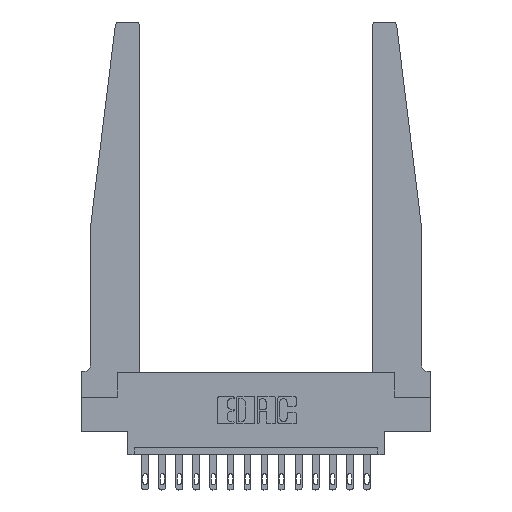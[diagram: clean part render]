
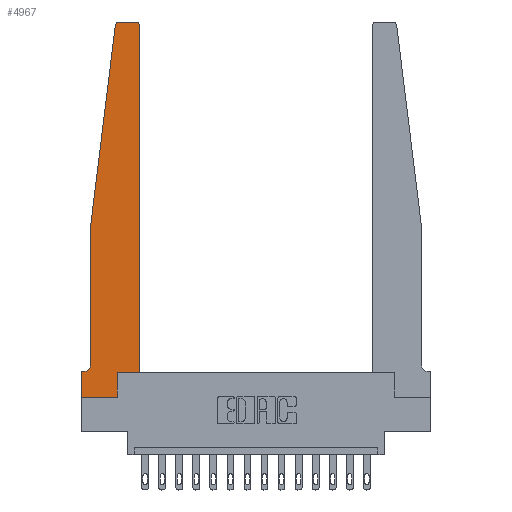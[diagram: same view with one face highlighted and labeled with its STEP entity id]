
A CAD part, top view. The second image highlights one B-rep face of the part: STEP entity #4967.
In plain terms, the highlighted planar face has unit normal (0, 0, 1).
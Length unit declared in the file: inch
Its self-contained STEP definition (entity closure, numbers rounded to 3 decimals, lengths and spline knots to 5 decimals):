
#178 = VERTEX_POINT ( 'NONE', #15564 ) ;
#372 = VERTEX_POINT ( 'NONE', #8095 ) ;
#437 = VERTEX_POINT ( 'NONE', #2567 ) ;
#461 = VERTEX_POINT ( 'NONE', #17534 ) ;
#1081 = VECTOR ( 'NONE', #7039, 39.37008 ) ;
#1116 = EDGE_CURVE ( 'NONE', #6186, #15797, #12551, .T. ) ;
#1315 = CARTESIAN_POINT ( 'NONE',  ( 0.015, 0.2375, 0.37 ) ) ;
#1372 = CARTESIAN_POINT ( 'NONE',  ( 0., 0., 0.37 ) ) ;
#1533 = ORIENTED_EDGE ( 'NONE', *, *, #12588, .T. ) ;
#1558 = DIRECTION ( 'NONE',  ( 0., -1., 0. ) ) ;
#1719 = VECTOR ( 'NONE', #12157, 39.37008 ) ;
#2425 = VERTEX_POINT ( 'NONE', #6968 ) ;
#2567 = CARTESIAN_POINT ( 'NONE',  ( 0.065, 1.25, 0.37 ) ) ;
#2598 = AXIS2_PLACEMENT_3D ( 'NONE', #13677, #2856, #17561 ) ;
#2856 = DIRECTION ( 'NONE',  ( 0., 0., 1. ) ) ;
#2908 = ORIENTED_EDGE ( 'NONE', *, *, #3953, .T. ) ;
#2912 = CARTESIAN_POINT ( 'NONE',  ( 0.395, 2.72, 0.37 ) ) ;
#2923 = DIRECTION ( 'NONE',  ( 0., 0., -1. ) ) ;
#2961 = EDGE_CURVE ( 'NONE', #10690, #16546, #6983, .T. ) ;
#3179 = VECTOR ( 'NONE', #1558, 39.37008 ) ;
#3345 = CARTESIAN_POINT ( 'NONE',  ( 0., 0., 0.37 ) ) ;
#3458 = VECTOR ( 'NONE', #15528, 39.37008 ) ;
#3953 = EDGE_CURVE ( 'NONE', #2425, #178, #16404, .T. ) ;
#4570 = CARTESIAN_POINT ( 'NONE',  ( 0., 0.1875, 0.37 ) ) ;
#4571 = EDGE_CURVE ( 'NONE', #437, #461, #13076, .T. ) ;
#4758 = EDGE_CURVE ( 'NONE', #12290, #11077, #11020, .T. ) ;
#4967 = ADVANCED_FACE ( 'NONE', ( #6512 ), #10468, .T. ) ;
#5254 = ORIENTED_EDGE ( 'NONE', *, *, #13176, .T. ) ;
#5280 = CARTESIAN_POINT ( 'NONE',  ( 0., 0.1875, 0.37 ) ) ;
#5446 = AXIS2_PLACEMENT_3D ( 'NONE', #5280, #10382, #9026 ) ;
#5924 = EDGE_LOOP ( 'NONE', ( #12108, #15944, #1533, #17374, #13289, #5254, #8734, #6416, #2908, #10328, #7662, #10372 ) ) ;
#6150 = CARTESIAN_POINT ( 'NONE',  ( 0.395, 2.75, 0.37 ) ) ;
#6186 = VERTEX_POINT ( 'NONE', #10662 ) ;
#6416 = ORIENTED_EDGE ( 'NONE', *, *, #7747, .T. ) ;
#6512 = FACE_OUTER_BOUND ( 'NONE', #5924, .T. ) ;
#6644 = DIRECTION ( 'NONE',  ( -1., 0., 0. ) ) ;
#6800 = VECTOR ( 'NONE', #15954, 39.37008 ) ;
#6968 = CARTESIAN_POINT ( 'NONE',  ( 0.2605, 0., 0.37 ) ) ;
#6983 = CIRCLE ( 'NONE', #17050, 0.03 ) ;
#6995 = EDGE_CURVE ( 'NONE', #16546, #6186, #8730, .T. ) ;
#7039 = DIRECTION ( 'NONE',  ( 0., 1., 0. ) ) ;
#7467 = CARTESIAN_POINT ( 'NONE',  ( 0.425, 0.18, 0.37 ) ) ;
#7662 = ORIENTED_EDGE ( 'NONE', *, *, #9104, .T. ) ;
#7747 = EDGE_CURVE ( 'NONE', #11077, #2425, #14326, .T. ) ;
#8095 = CARTESIAN_POINT ( 'NONE',  ( 0.015, 0.1875, 0.37 ) ) ;
#8730 = LINE ( 'NONE', #17008, #11979 ) ;
#8734 = ORIENTED_EDGE ( 'NONE', *, *, #4758, .T. ) ;
#9026 = DIRECTION ( 'NONE',  ( 1., 0., 0. ) ) ;
#9104 = EDGE_CURVE ( 'NONE', #15228, #10690, #15219, .T. ) ;
#9974 = VECTOR ( 'NONE', #13397, 39.37008 ) ;
#10060 = DIRECTION ( 'NONE',  ( -0.122, -0.992, 0. ) ) ;
#10076 = CARTESIAN_POINT ( 'NONE',  ( 0., 0., 0.37 ) ) ;
#10172 = CARTESIAN_POINT ( 'NONE',  ( 0.425, 2.72, 0.37 ) ) ;
#10328 = ORIENTED_EDGE ( 'NONE', *, *, #14896, .T. ) ;
#10372 = ORIENTED_EDGE ( 'NONE', *, *, #2961, .T. ) ;
#10382 = DIRECTION ( 'NONE',  ( 0., 0., 1. ) ) ;
#10468 = PLANE ( 'NONE',  #5446 ) ;
#10531 = AXIS2_PLACEMENT_3D ( 'NONE', #1315, #2923, #6644 ) ;
#10598 = VECTOR ( 'NONE', #15415, 39.37008 ) ;
#10662 = CARTESIAN_POINT ( 'NONE',  ( 0.27653, 2.75, 0.37 ) ) ;
#10690 = VERTEX_POINT ( 'NONE', #10172 ) ;
#11009 = CARTESIAN_POINT ( 'NONE',  ( 0.425, 0.18, 0.37 ) ) ;
#11020 = LINE ( 'NONE', #1372, #3179 ) ;
#11077 = VERTEX_POINT ( 'NONE', #10076 ) ;
#11326 = EDGE_CURVE ( 'NONE', #461, #372, #12232, .T. ) ;
#11827 = CARTESIAN_POINT ( 'NONE',  ( 0.065, 0.1875, 0.37 ) ) ;
#11979 = VECTOR ( 'NONE', #14196, 39.37008 ) ;
#12108 = ORIENTED_EDGE ( 'NONE', *, *, #6995, .T. ) ;
#12157 = DIRECTION ( 'NONE',  ( 0., 1., 0. ) ) ;
#12172 = CARTESIAN_POINT ( 'NONE',  ( 0.24675, 2.72367, 0.37 ) ) ;
#12232 = CIRCLE ( 'NONE', #10531, 0.05 ) ;
#12290 = VERTEX_POINT ( 'NONE', #4570 ) ;
#12551 = CIRCLE ( 'NONE', #2598, 0.03 ) ;
#12554 = DIRECTION ( 'NONE',  ( 0., 0., 1. ) ) ;
#12588 = EDGE_CURVE ( 'NONE', #15797, #437, #14176, .T. ) ;
#13076 = LINE ( 'NONE', #17237, #3458 ) ;
#13142 = LINE ( 'NONE', #17373, #9974 ) ;
#13176 = EDGE_CURVE ( 'NONE', #372, #12290, #17048, .T. ) ;
#13289 = ORIENTED_EDGE ( 'NONE', *, *, #11326, .T. ) ;
#13397 = DIRECTION ( 'NONE',  ( 1., 0., 0. ) ) ;
#13503 = CARTESIAN_POINT ( 'NONE',  ( 0.2605, 0.18, 0.37 ) ) ;
#13677 = CARTESIAN_POINT ( 'NONE',  ( 0.27653, 2.72, 0.37 ) ) ;
#14001 = CARTESIAN_POINT ( 'NONE',  ( 0.065, 1.25, 0.37 ) ) ;
#14176 = LINE ( 'NONE', #14001, #17412 ) ;
#14196 = DIRECTION ( 'NONE',  ( -1., 0., 0. ) ) ;
#14326 = LINE ( 'NONE', #3345, #10598 ) ;
#14896 = EDGE_CURVE ( 'NONE', #178, #15228, #13142, .T. ) ;
#15219 = LINE ( 'NONE', #11009, #1081 ) ;
#15228 = VERTEX_POINT ( 'NONE', #7467 ) ;
#15415 = DIRECTION ( 'NONE',  ( 1., 0., 0. ) ) ;
#15528 = DIRECTION ( 'NONE',  ( 0., -1., 0. ) ) ;
#15564 = CARTESIAN_POINT ( 'NONE',  ( 0.2605, 0.18, 0.37 ) ) ;
#15797 = VERTEX_POINT ( 'NONE', #12172 ) ;
#15944 = ORIENTED_EDGE ( 'NONE', *, *, #1116, .T. ) ;
#15954 = DIRECTION ( 'NONE',  ( -1., 0., 0. ) ) ;
#16404 = LINE ( 'NONE', #13503, #1719 ) ;
#16522 = DIRECTION ( 'NONE',  ( 1., 0., 0. ) ) ;
#16546 = VERTEX_POINT ( 'NONE', #6150 ) ;
#17008 = CARTESIAN_POINT ( 'NONE',  ( 0.25, 2.75, 0.37 ) ) ;
#17048 = LINE ( 'NONE', #11827, #6800 ) ;
#17050 = AXIS2_PLACEMENT_3D ( 'NONE', #2912, #12554, #16522 ) ;
#17237 = CARTESIAN_POINT ( 'NONE',  ( 0.065, 1.25, 0.37 ) ) ;
#17373 = CARTESIAN_POINT ( 'NONE',  ( 0.425, 0.18, 0.37 ) ) ;
#17374 = ORIENTED_EDGE ( 'NONE', *, *, #4571, .T. ) ;
#17412 = VECTOR ( 'NONE', #10060, 39.37008 ) ;
#17534 = CARTESIAN_POINT ( 'NONE',  ( 0.065, 0.2375, 0.37 ) ) ;
#17561 = DIRECTION ( 'NONE',  ( 1., 0., 0. ) ) ;
